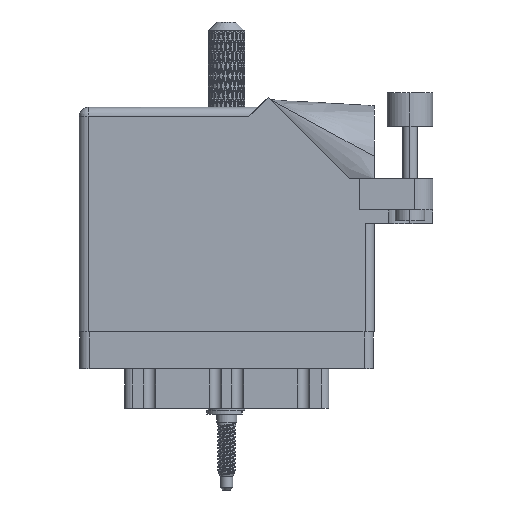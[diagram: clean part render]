
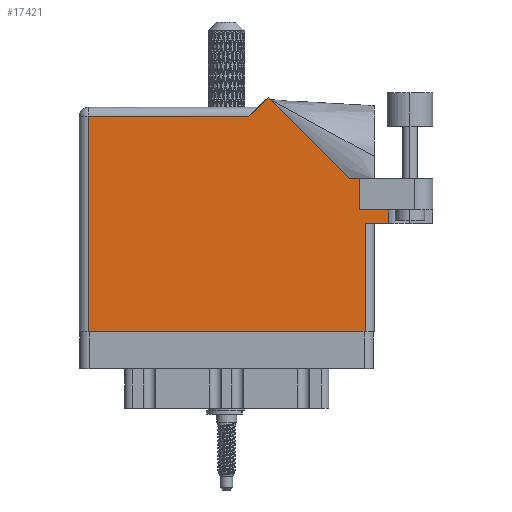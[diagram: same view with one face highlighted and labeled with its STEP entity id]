
A CAD part, front view. The second image highlights one B-rep face of the part: STEP entity #17421.
In plain terms, the highlighted face is planar.
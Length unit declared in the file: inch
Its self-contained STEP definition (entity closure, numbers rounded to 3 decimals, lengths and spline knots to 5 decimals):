
#686 = ORIENTED_EDGE ( 'NONE', *, *, #21397, .T. ) ;
#951 = CARTESIAN_POINT ( 'NONE',  ( 1.948, 0., 0. ) ) ;
#1313 = ORIENTED_EDGE ( 'NONE', *, *, #73740, .T. ) ;
#1467 = VERTEX_POINT ( 'NONE', #52377 ) ;
#1728 = ORIENTED_EDGE ( 'NONE', *, *, #10668, .T. ) ;
#2568 = CARTESIAN_POINT ( 'NONE',  ( 1.84442, 1.044, 0. ) ) ;
#2972 = VECTOR ( 'NONE', #95300, 39.37008 ) ;
#4371 = VERTEX_POINT ( 'NONE', #21204 ) ;
#4791 = DIRECTION ( 'NONE',  ( 1., 0., 0. ) ) ;
#4865 = ORIENTED_EDGE ( 'NONE', *, *, #43205, .T. ) ;
#5346 = LINE ( 'NONE', #78512, #33994 ) ;
#7767 = VECTOR ( 'NONE', #62393, 39.37008 ) ;
#9381 = DIRECTION ( 'NONE',  ( -1., 0., 0. ) ) ;
#10081 = VECTOR ( 'NONE', #45296, 39.37008 ) ;
#10668 = EDGE_CURVE ( 'NONE', #4371, #17865, #60267, .T. ) ;
#12444 = CARTESIAN_POINT ( 'NONE',  ( 0.062, 0., 0. ) ) ;
#13574 = VECTOR ( 'NONE', #44836, 39.37008 ) ;
#15651 = LINE ( 'NONE', #71863, #74702 ) ;
#16251 = LINE ( 'NONE', #25269, #64700 ) ;
#17421 = ADVANCED_FACE ( 'NONE', ( #98914 ), #26297, .F. ) ;
#17865 = VERTEX_POINT ( 'NONE', #73374 ) ;
#18868 = CARTESIAN_POINT ( 'NONE',  ( 2.1115, 0.831, 0. ) ) ;
#19762 = VERTEX_POINT ( 'NONE', #84126 ) ;
#21204 = CARTESIAN_POINT ( 'NONE',  ( 1.155, 1.468, 0. ) ) ;
#21397 = EDGE_CURVE ( 'NONE', #38072, #1467, #53988, .T. ) ;
#22117 = ORIENTED_EDGE ( 'NONE', *, *, #68166, .T. ) ;
#23868 = DIRECTION ( 'NONE',  ( 1., 0., 0. ) ) ;
#25269 = CARTESIAN_POINT ( 'NONE',  ( 2.1115, 1.16177, 0. ) ) ;
#25590 = LINE ( 'NONE', #35136, #30920 ) ;
#26297 = PLANE ( 'NONE',  #29494 ) ;
#27301 = LINE ( 'NONE', #12444, #13574 ) ;
#27394 = ORIENTED_EDGE ( 'NONE', *, *, #82563, .T. ) ;
#27779 = CARTESIAN_POINT ( 'NONE',  ( 1.91, 0.831, 0. ) ) ;
#28231 = EDGE_CURVE ( 'NONE', #33981, #19762, #16251, .T. ) ;
#28464 = LINE ( 'NONE', #60836, #7767 ) ;
#29385 = DIRECTION ( 'NONE',  ( -0.707, -0.707, 0. ) ) ;
#29494 = AXIS2_PLACEMENT_3D ( 'NONE', #85146, #50712, #83562 ) ;
#29955 = EDGE_LOOP ( 'NONE', ( #22117, #32277, #1313, #86576, #81638, #4865, #57188, #686, #27394, #1728, #90669 ) ) ;
#30120 = EDGE_CURVE ( 'NONE', #63551, #38072, #25590, .T. ) ;
#30920 = VECTOR ( 'NONE', #83364, 39.37008 ) ;
#32277 = ORIENTED_EDGE ( 'NONE', *, *, #100935, .T. ) ;
#33981 = VERTEX_POINT ( 'NONE', #18868 ) ;
#33994 = VECTOR ( 'NONE', #4791, 39.37008 ) ;
#35136 = CARTESIAN_POINT ( 'NONE',  ( 2.41, 1.044, 0. ) ) ;
#37365 = LINE ( 'NONE', #27779, #10081 ) ;
#38072 = VERTEX_POINT ( 'NONE', #2568 ) ;
#43205 = EDGE_CURVE ( 'NONE', #64537, #63551, #37365, .T. ) ;
#44836 = DIRECTION ( 'NONE',  ( 0., -1., 0. ) ) ;
#45296 = DIRECTION ( 'NONE',  ( 0., 1., 0. ) ) ;
#48192 = EDGE_CURVE ( 'NONE', #17865, #62540, #27301, .T. ) ;
#49321 = CARTESIAN_POINT ( 'NONE',  ( 1.91, 0.831, 0. ) ) ;
#49799 = CARTESIAN_POINT ( 'NONE',  ( 0.062, 0., 0. ) ) ;
#50712 = DIRECTION ( 'NONE',  ( 0., 0., -1. ) ) ;
#52377 = CARTESIAN_POINT ( 'NONE',  ( 1.28771, 1.60071, 0. ) ) ;
#53988 = LINE ( 'NONE', #62471, #2972 ) ;
#57188 = ORIENTED_EDGE ( 'NONE', *, *, #30120, .T. ) ;
#60267 = LINE ( 'NONE', #92567, #98065 ) ;
#60836 = CARTESIAN_POINT ( 'NONE',  ( 1.948, 0.737, 0. ) ) ;
#61228 = LINE ( 'NONE', #68618, #88016 ) ;
#62393 = DIRECTION ( 'NONE',  ( 0., 1., 0. ) ) ;
#62471 = CARTESIAN_POINT ( 'NONE',  ( 1.84442, 1.044, 0. ) ) ;
#62540 = VERTEX_POINT ( 'NONE', #49799 ) ;
#63551 = VERTEX_POINT ( 'NONE', #65197 ) ;
#64174 = CARTESIAN_POINT ( 'NONE',  ( 2.01, 0.737, 0. ) ) ;
#64537 = VERTEX_POINT ( 'NONE', #49321 ) ;
#64700 = VECTOR ( 'NONE', #89964, 39.37008 ) ;
#65197 = CARTESIAN_POINT ( 'NONE',  ( 1.91, 1.044, 0. ) ) ;
#68166 = EDGE_CURVE ( 'NONE', #62540, #79622, #15651, .T. ) ;
#68618 = CARTESIAN_POINT ( 'NONE',  ( 1.217, 1.53, 0. ) ) ;
#71863 = CARTESIAN_POINT ( 'NONE',  ( 0., 0., 0. ) ) ;
#72094 = LINE ( 'NONE', #64174, #72640 ) ;
#72640 = VECTOR ( 'NONE', #23868, 39.37008 ) ;
#73374 = CARTESIAN_POINT ( 'NONE',  ( 0.062, 1.468, 0. ) ) ;
#73740 = EDGE_CURVE ( 'NONE', #77028, #19762, #72094, .T. ) ;
#74702 = VECTOR ( 'NONE', #81923, 39.37008 ) ;
#77028 = VERTEX_POINT ( 'NONE', #104583 ) ;
#78512 = CARTESIAN_POINT ( 'NONE',  ( 1.91, 0.831, 0. ) ) ;
#79622 = VERTEX_POINT ( 'NONE', #951 ) ;
#81638 = ORIENTED_EDGE ( 'NONE', *, *, #84922, .F. ) ;
#81923 = DIRECTION ( 'NONE',  ( 1., 0., 0. ) ) ;
#82563 = EDGE_CURVE ( 'NONE', #1467, #4371, #61228, .T. ) ;
#83364 = DIRECTION ( 'NONE',  ( -1., 0., 0. ) ) ;
#83562 = DIRECTION ( 'NONE',  ( -1., 0., 0. ) ) ;
#84126 = CARTESIAN_POINT ( 'NONE',  ( 2.1115, 0.737, 0. ) ) ;
#84922 = EDGE_CURVE ( 'NONE', #64537, #33981, #5346, .T. ) ;
#85146 = CARTESIAN_POINT ( 'NONE',  ( 0., 1.53, 0. ) ) ;
#86576 = ORIENTED_EDGE ( 'NONE', *, *, #28231, .F. ) ;
#88016 = VECTOR ( 'NONE', #29385, 39.37008 ) ;
#89964 = DIRECTION ( 'NONE',  ( 0., -1., 0. ) ) ;
#90669 = ORIENTED_EDGE ( 'NONE', *, *, #48192, .T. ) ;
#92567 = CARTESIAN_POINT ( 'NONE',  ( 0., 1.468, 0. ) ) ;
#95300 = DIRECTION ( 'NONE',  ( -0.707, 0.707, 0. ) ) ;
#98065 = VECTOR ( 'NONE', #9381, 39.37008 ) ;
#98914 = FACE_OUTER_BOUND ( 'NONE', #29955, .T. ) ;
#100935 = EDGE_CURVE ( 'NONE', #79622, #77028, #28464, .T. ) ;
#104583 = CARTESIAN_POINT ( 'NONE',  ( 1.948, 0.737, 0. ) ) ;
